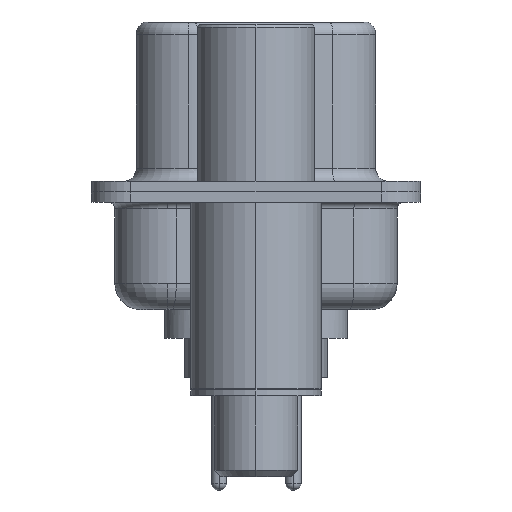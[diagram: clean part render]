
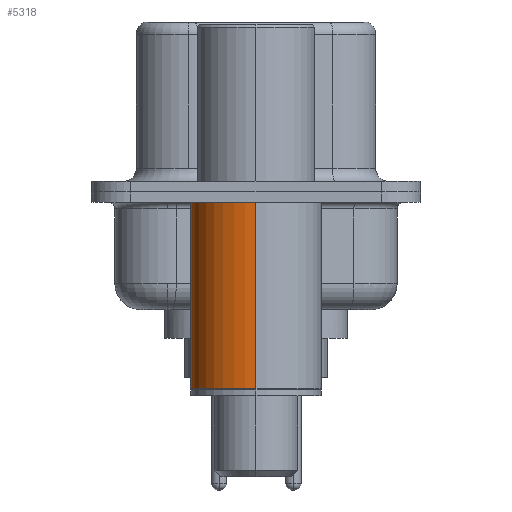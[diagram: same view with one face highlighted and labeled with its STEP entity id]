
A CAD part, left-side view. The second image highlights one B-rep face of the part: STEP entity #5318.
In plain terms, the highlighted cylindrical face has radius 2.5 mm (diameter 5 mm), a partial arc.
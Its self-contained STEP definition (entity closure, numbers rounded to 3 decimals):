
#235 = CARTESIAN_POINT ( 'NONE',  ( -2.5, 0., 0.581 ) ) ;
#350 = AXIS2_PLACEMENT_3D ( 'NONE', #16053, #7250, #17535 ) ;
#3600 = CYLINDRICAL_SURFACE ( 'NONE', #5819, 2.5 ) ;
#3656 = DIRECTION ( 'NONE',  ( 0., 0., 1. ) ) ;
#4022 = DIRECTION ( 'NONE',  ( 1., 0., 0. ) ) ;
#4144 = CARTESIAN_POINT ( 'NONE',  ( -2.5, 0., -7.525 ) ) ;
#4461 = EDGE_CURVE ( 'NONE', #6646, #10147, #15585, .T. ) ;
#5318 = ADVANCED_FACE ( 'NONE', ( #15328 ), #3600, .T. ) ;
#5819 = AXIS2_PLACEMENT_3D ( 'NONE', #15501, #13847, #11051 ) ;
#6152 = CARTESIAN_POINT ( 'NONE',  ( 0., 0., -7.525 ) ) ;
#6646 = VERTEX_POINT ( 'NONE', #13960 ) ;
#7250 = DIRECTION ( 'NONE',  ( 0., 0., 1. ) ) ;
#8793 = VECTOR ( 'NONE', #16438, 1000. ) ;
#9026 = DIRECTION ( 'NONE',  ( 0., 0., 1. ) ) ;
#9457 = VERTEX_POINT ( 'NONE', #12800 ) ;
#10147 = VERTEX_POINT ( 'NONE', #4144 ) ;
#10682 = AXIS2_PLACEMENT_3D ( 'NONE', #6152, #3656, #4022 ) ;
#10877 = VECTOR ( 'NONE', #9026, 1000. ) ;
#11051 = DIRECTION ( 'NONE',  ( 1., 0., 0. ) ) ;
#11196 = EDGE_LOOP ( 'NONE', ( #18821, #17729, #13804, #14737 ) ) ;
#11327 = LINE ( 'NONE', #235, #10877 ) ;
#12365 = CARTESIAN_POINT ( 'NONE',  ( -2.5, 0., -0.4 ) ) ;
#12565 = EDGE_CURVE ( 'NONE', #9457, #13726, #15450, .T. ) ;
#12708 = EDGE_CURVE ( 'NONE', #6646, #9457, #16608, .T. ) ;
#12800 = CARTESIAN_POINT ( 'NONE',  ( 2.5, 0., -0.4 ) ) ;
#13304 = EDGE_CURVE ( 'NONE', #10147, #13726, #11327, .T. ) ;
#13726 = VERTEX_POINT ( 'NONE', #12365 ) ;
#13804 = ORIENTED_EDGE ( 'NONE', *, *, #12565, .F. ) ;
#13847 = DIRECTION ( 'NONE',  ( 0., 0., 1. ) ) ;
#13960 = CARTESIAN_POINT ( 'NONE',  ( 2.5, 0., -7.525 ) ) ;
#14737 = ORIENTED_EDGE ( 'NONE', *, *, #12708, .F. ) ;
#15018 = CARTESIAN_POINT ( 'NONE',  ( 2.5, 0., 0.581 ) ) ;
#15328 = FACE_OUTER_BOUND ( 'NONE', #11196, .T. ) ;
#15450 = CIRCLE ( 'NONE', #350, 2.5 ) ;
#15501 = CARTESIAN_POINT ( 'NONE',  ( 0., 0., 0.581 ) ) ;
#15585 = CIRCLE ( 'NONE', #10682, 2.5 ) ;
#16053 = CARTESIAN_POINT ( 'NONE',  ( 0., 0., -0.4 ) ) ;
#16438 = DIRECTION ( 'NONE',  ( 0., 0., 1. ) ) ;
#16608 = LINE ( 'NONE', #15018, #8793 ) ;
#17535 = DIRECTION ( 'NONE',  ( 1., 0., 0. ) ) ;
#17729 = ORIENTED_EDGE ( 'NONE', *, *, #13304, .T. ) ;
#18821 = ORIENTED_EDGE ( 'NONE', *, *, #4461, .T. ) ;
